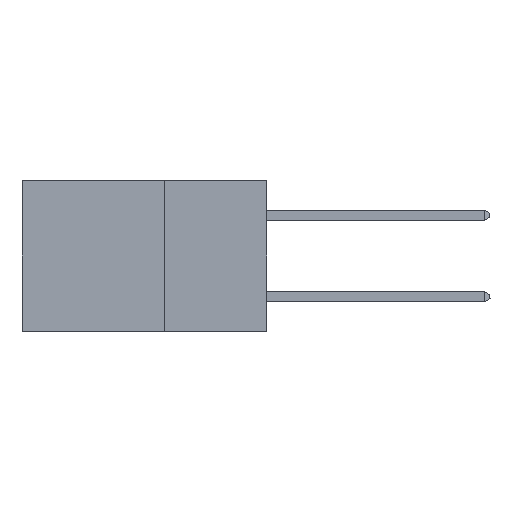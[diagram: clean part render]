
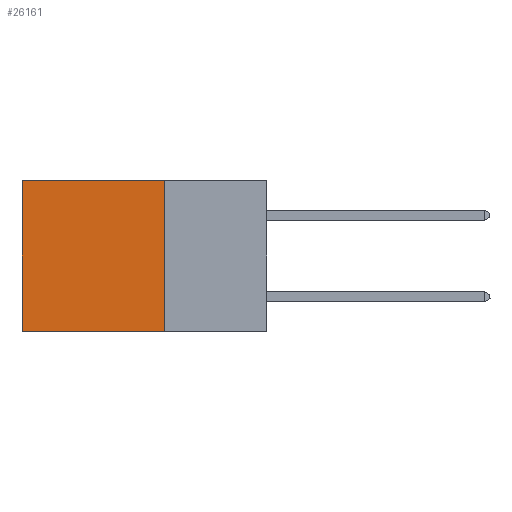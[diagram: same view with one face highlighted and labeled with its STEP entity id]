
A CAD part, left-side view. The second image highlights one B-rep face of the part: STEP entity #26161.
In plain terms, the highlighted planar face has unit normal (-1, 0, 0).
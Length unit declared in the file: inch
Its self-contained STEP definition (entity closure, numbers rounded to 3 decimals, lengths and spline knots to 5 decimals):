
#152 = LINE ( 'NONE', #13611, #24770 ) ;
#230 = EDGE_CURVE ( 'NONE', #5763, #27069, #7779, .T. ) ;
#291 = EDGE_CURVE ( 'NONE', #27995, #27069, #26387, .T. ) ;
#391 = ORIENTED_EDGE ( 'NONE', *, *, #291, .F. ) ;
#1065 = ORIENTED_EDGE ( 'NONE', *, *, #230, .T. ) ;
#2854 = EDGE_CURVE ( 'NONE', #4695, #27995, #152, .T. ) ;
#4695 = VERTEX_POINT ( 'NONE', #28804 ) ;
#5232 = VECTOR ( 'NONE', #17903, 39.37008 ) ;
#5763 = VERTEX_POINT ( 'NONE', #9164 ) ;
#6549 = CARTESIAN_POINT ( 'NONE',  ( 0.2875, 0.25, -0.37 ) ) ;
#7779 = LINE ( 'NONE', #16500, #21206 ) ;
#8287 = EDGE_LOOP ( 'NONE', ( #1065, #391, #23282, #13489 ) ) ;
#8844 = VECTOR ( 'NONE', #21358, 39.37008 ) ;
#9164 = CARTESIAN_POINT ( 'NONE',  ( 0.2875, 0.6, 0. ) ) ;
#9300 = AXIS2_PLACEMENT_3D ( 'NONE', #16264, #14128, #11956 ) ;
#9464 = FACE_OUTER_BOUND ( 'NONE', #8287, .T. ) ;
#11153 = DIRECTION ( 'NONE',  ( 0., 0., -1. ) ) ;
#11902 = DIRECTION ( 'NONE',  ( 0., 0., -1. ) ) ;
#11956 = DIRECTION ( 'NONE',  ( 0., 0., -1. ) ) ;
#13489 = ORIENTED_EDGE ( 'NONE', *, *, #14745, .T. ) ;
#13611 = CARTESIAN_POINT ( 'NONE',  ( 0.2875, 0.25, 0. ) ) ;
#14128 = DIRECTION ( 'NONE',  ( 1., 0., 0. ) ) ;
#14745 = EDGE_CURVE ( 'NONE', #4695, #5763, #15767, .T. ) ;
#15767 = LINE ( 'NONE', #22528, #5232 ) ;
#16264 = CARTESIAN_POINT ( 'NONE',  ( 0.2875, 0.25, 0. ) ) ;
#16500 = CARTESIAN_POINT ( 'NONE',  ( 0.2875, 0.6, 0. ) ) ;
#17903 = DIRECTION ( 'NONE',  ( 0., 1., 0. ) ) ;
#18654 = PLANE ( 'NONE',  #9300 ) ;
#20962 = CARTESIAN_POINT ( 'NONE',  ( 0.2875, 0.25, -0.37 ) ) ;
#21206 = VECTOR ( 'NONE', #11902, 39.37008 ) ;
#21358 = DIRECTION ( 'NONE',  ( 0., 1., 0. ) ) ;
#21386 = CARTESIAN_POINT ( 'NONE',  ( 0.2875, 0.6, -0.37 ) ) ;
#22528 = CARTESIAN_POINT ( 'NONE',  ( 0.2875, 0.25, 0. ) ) ;
#23282 = ORIENTED_EDGE ( 'NONE', *, *, #2854, .F. ) ;
#24770 = VECTOR ( 'NONE', #11153, 39.37008 ) ;
#26161 = ADVANCED_FACE ( 'NONE', ( #9464 ), #18654, .F. ) ;
#26387 = LINE ( 'NONE', #20962, #8844 ) ;
#27069 = VERTEX_POINT ( 'NONE', #21386 ) ;
#27995 = VERTEX_POINT ( 'NONE', #6549 ) ;
#28804 = CARTESIAN_POINT ( 'NONE',  ( 0.2875, 0.25, 0. ) ) ;
